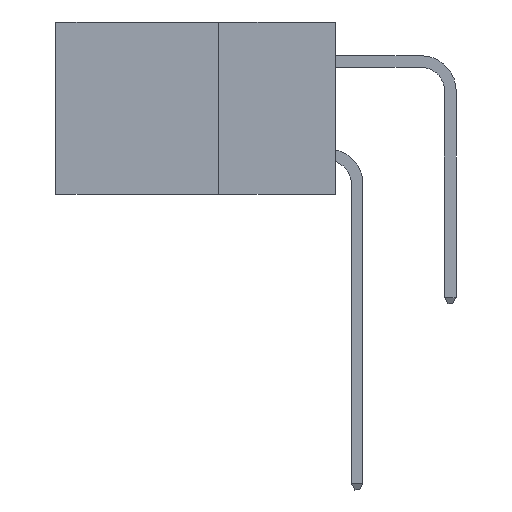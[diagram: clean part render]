
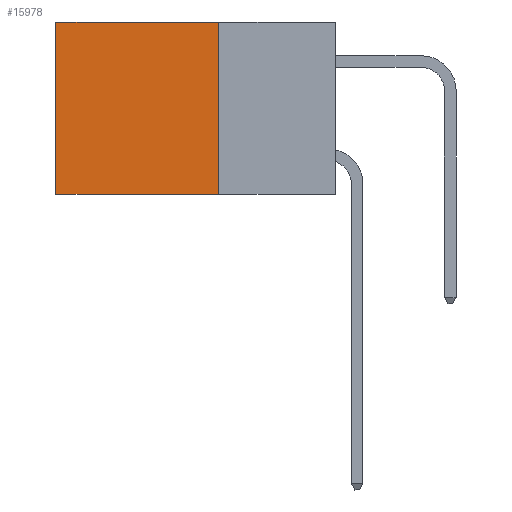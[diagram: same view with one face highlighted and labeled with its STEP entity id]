
A CAD part, left-side view. The second image highlights one B-rep face of the part: STEP entity #15978.
In plain terms, the highlighted planar face has unit normal (-1, 0, 0).
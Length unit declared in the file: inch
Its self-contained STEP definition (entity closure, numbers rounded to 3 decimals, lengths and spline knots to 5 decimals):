
#758 = CARTESIAN_POINT ( 'NONE',  ( 0.2875, 0.6, 0. ) ) ;
#1351 = EDGE_CURVE ( 'NONE', #7892, #17781, #11175, .T. ) ;
#1421 = CARTESIAN_POINT ( 'NONE',  ( 0.2875, 0.25, -0.37 ) ) ;
#2001 = DIRECTION ( 'NONE',  ( 0., 0., -1. ) ) ;
#2319 = EDGE_CURVE ( 'NONE', #7892, #9426, #12129, .T. ) ;
#2653 = DIRECTION ( 'NONE',  ( 0., 1., 0. ) ) ;
#3259 = CARTESIAN_POINT ( 'NONE',  ( 0.2875, 0.25, 0. ) ) ;
#4294 = VECTOR ( 'NONE', #5402, 39.37008 ) ;
#5402 = DIRECTION ( 'NONE',  ( 0., 0., -1. ) ) ;
#5800 = VERTEX_POINT ( 'NONE', #16791 ) ;
#5941 = EDGE_CURVE ( 'NONE', #17781, #5800, #17693, .T. ) ;
#6359 = VECTOR ( 'NONE', #2653, 39.37008 ) ;
#6851 = VECTOR ( 'NONE', #11133, 39.37008 ) ;
#7892 = VERTEX_POINT ( 'NONE', #15086 ) ;
#7984 = CARTESIAN_POINT ( 'NONE',  ( 0.2875, 0.25, -0.37 ) ) ;
#8177 = LINE ( 'NONE', #1421, #6359 ) ;
#8207 = CARTESIAN_POINT ( 'NONE',  ( 0.2875, 0.25, 0. ) ) ;
#9276 = PLANE ( 'NONE',  #9530 ) ;
#9426 = VERTEX_POINT ( 'NONE', #7984 ) ;
#9530 = AXIS2_PLACEMENT_3D ( 'NONE', #3259, #10735, #2001 ) ;
#9627 = ORIENTED_EDGE ( 'NONE', *, *, #5941, .T. ) ;
#10735 = DIRECTION ( 'NONE',  ( 1., 0., 0. ) ) ;
#11133 = DIRECTION ( 'NONE',  ( 0., 1., 0. ) ) ;
#11175 = LINE ( 'NONE', #18486, #6851 ) ;
#11286 = DIRECTION ( 'NONE',  ( 0., 0., -1. ) ) ;
#12129 = LINE ( 'NONE', #8207, #4294 ) ;
#12701 = FACE_OUTER_BOUND ( 'NONE', #13116, .T. ) ;
#13081 = ORIENTED_EDGE ( 'NONE', *, *, #1351, .T. ) ;
#13116 = EDGE_LOOP ( 'NONE', ( #9627, #17798, #14248, #13081 ) ) ;
#13352 = VECTOR ( 'NONE', #11286, 39.37008 ) ;
#14215 = EDGE_CURVE ( 'NONE', #9426, #5800, #8177, .T. ) ;
#14248 = ORIENTED_EDGE ( 'NONE', *, *, #2319, .F. ) ;
#15086 = CARTESIAN_POINT ( 'NONE',  ( 0.2875, 0.25, 0. ) ) ;
#15747 = CARTESIAN_POINT ( 'NONE',  ( 0.2875, 0.6, 0. ) ) ;
#15978 = ADVANCED_FACE ( 'NONE', ( #12701 ), #9276, .F. ) ;
#16791 = CARTESIAN_POINT ( 'NONE',  ( 0.2875, 0.6, -0.37 ) ) ;
#17693 = LINE ( 'NONE', #15747, #13352 ) ;
#17781 = VERTEX_POINT ( 'NONE', #758 ) ;
#17798 = ORIENTED_EDGE ( 'NONE', *, *, #14215, .F. ) ;
#18486 = CARTESIAN_POINT ( 'NONE',  ( 0.2875, 0.25, 0. ) ) ;
